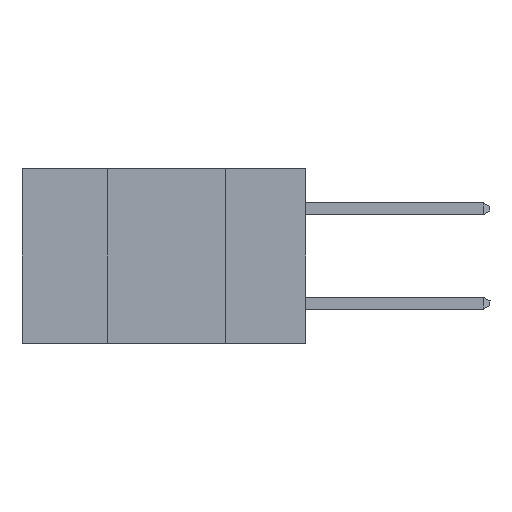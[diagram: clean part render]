
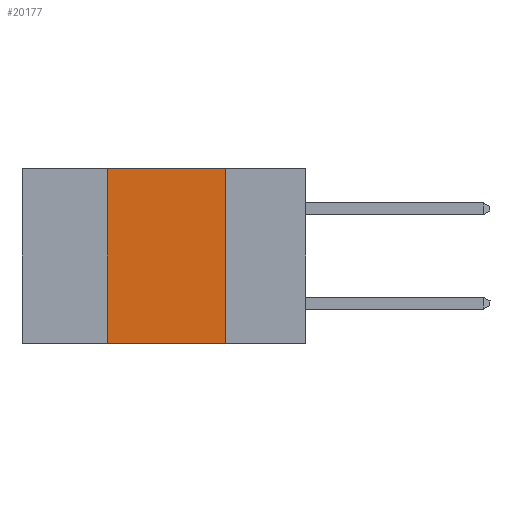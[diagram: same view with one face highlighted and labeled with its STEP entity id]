
A CAD part, left-side view. The second image highlights one B-rep face of the part: STEP entity #20177.
In plain terms, the highlighted planar face has unit normal (-1, 0, 0).
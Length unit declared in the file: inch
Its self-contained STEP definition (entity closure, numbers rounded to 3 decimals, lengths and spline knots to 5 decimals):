
#496 = DIRECTION ( 'NONE',  ( 0., -1., 0. ) ) ;
#560 = EDGE_CURVE ( 'NONE', #9003, #19377, #6858, .T. ) ;
#623 = CARTESIAN_POINT ( 'NONE',  ( 0., 0.6, 0. ) ) ;
#720 = CARTESIAN_POINT ( 'NONE',  ( 0., 0.6, -0.37 ) ) ;
#733 = VERTEX_POINT ( 'NONE', #5344 ) ;
#1010 = DIRECTION ( 'NONE',  ( 1., 0., 0. ) ) ;
#1290 = VECTOR ( 'NONE', #7637, 39.37008 ) ;
#1886 = LINE ( 'NONE', #20299, #1290 ) ;
#2265 = EDGE_CURVE ( 'NONE', #19377, #733, #9106, .T. ) ;
#2582 = DIRECTION ( 'NONE',  ( 0., -1., 0. ) ) ;
#3740 = AXIS2_PLACEMENT_3D ( 'NONE', #12119, #1010, #13948 ) ;
#4137 = VECTOR ( 'NONE', #496, 39.37008 ) ;
#4596 = LINE ( 'NONE', #720, #13838 ) ;
#5209 = CARTESIAN_POINT ( 'NONE',  ( 0., 0.42, -0.37 ) ) ;
#5344 = CARTESIAN_POINT ( 'NONE',  ( 0., 0.17, 0. ) ) ;
#6858 = LINE ( 'NONE', #8534, #16024 ) ;
#7637 = DIRECTION ( 'NONE',  ( 0., 0., -1. ) ) ;
#7870 = ORIENTED_EDGE ( 'NONE', *, *, #10078, .T. ) ;
#8534 = CARTESIAN_POINT ( 'NONE',  ( 0., 0.42, -0.37 ) ) ;
#9003 = VERTEX_POINT ( 'NONE', #5209 ) ;
#9106 = LINE ( 'NONE', #623, #4137 ) ;
#10078 = EDGE_CURVE ( 'NONE', #9003, #19489, #4596, .T. ) ;
#10467 = ORIENTED_EDGE ( 'NONE', *, *, #21803, .F. ) ;
#10713 = EDGE_LOOP ( 'NONE', ( #10467, #11616, #16431, #7870 ) ) ;
#11616 = ORIENTED_EDGE ( 'NONE', *, *, #2265, .F. ) ;
#12119 = CARTESIAN_POINT ( 'NONE',  ( 0., 0.6, 0. ) ) ;
#13586 = CARTESIAN_POINT ( 'NONE',  ( 0., 0.42, 0. ) ) ;
#13838 = VECTOR ( 'NONE', #2582, 39.37008 ) ;
#13948 = DIRECTION ( 'NONE',  ( 0., 0., -1. ) ) ;
#16024 = VECTOR ( 'NONE', #16340, 39.37008 ) ;
#16340 = DIRECTION ( 'NONE',  ( 0., 0., 1. ) ) ;
#16431 = ORIENTED_EDGE ( 'NONE', *, *, #560, .F. ) ;
#19377 = VERTEX_POINT ( 'NONE', #13586 ) ;
#19489 = VERTEX_POINT ( 'NONE', #22798 ) ;
#20177 = ADVANCED_FACE ( 'NONE', ( #21418 ), #21046, .F. ) ;
#20299 = CARTESIAN_POINT ( 'NONE',  ( 0., 0.17, -0.37 ) ) ;
#21046 = PLANE ( 'NONE',  #3740 ) ;
#21418 = FACE_OUTER_BOUND ( 'NONE', #10713, .T. ) ;
#21803 = EDGE_CURVE ( 'NONE', #733, #19489, #1886, .T. ) ;
#22798 = CARTESIAN_POINT ( 'NONE',  ( 0., 0.17, -0.37 ) ) ;
